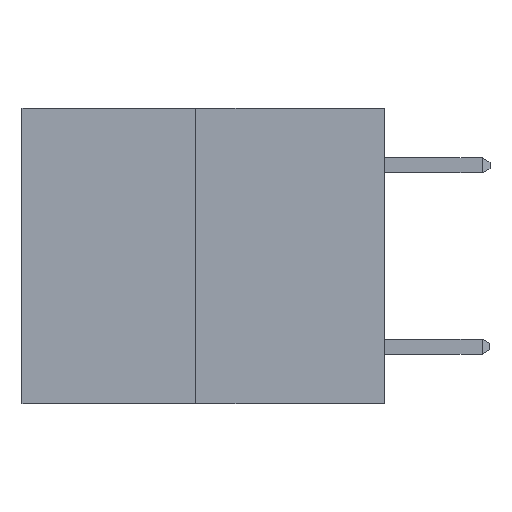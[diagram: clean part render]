
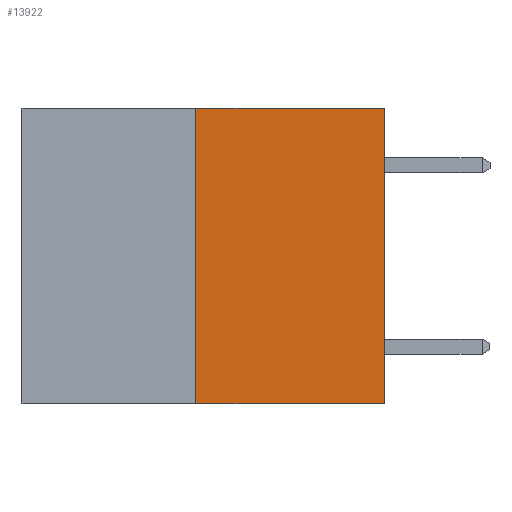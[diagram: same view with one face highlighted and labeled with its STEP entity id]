
A CAD part, left-side view. The second image highlights one B-rep face of the part: STEP entity #13922.
In plain terms, the highlighted planar face has unit normal (-1, 0, 0).
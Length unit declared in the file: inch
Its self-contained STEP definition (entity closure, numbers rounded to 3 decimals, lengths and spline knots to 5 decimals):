
#93 = DIRECTION ( 'NONE',  ( 0., -1., 0. ) ) ;
#161 = CARTESIAN_POINT ( 'NONE',  ( 0., 0.6, -0.49 ) ) ;
#312 = CARTESIAN_POINT ( 'NONE',  ( 0., 0., 0. ) ) ;
#816 = EDGE_CURVE ( 'NONE', #3410, #12007, #6694, .T. ) ;
#1347 = ORIENTED_EDGE ( 'NONE', *, *, #5956, .T. ) ;
#2114 = EDGE_CURVE ( 'NONE', #3410, #12522, #3185, .T. ) ;
#2272 = FACE_OUTER_BOUND ( 'NONE', #8951, .T. ) ;
#2341 = DIRECTION ( 'NONE',  ( 1., 0., 0. ) ) ;
#2649 = LINE ( 'NONE', #12723, #13413 ) ;
#2739 = ORIENTED_EDGE ( 'NONE', *, *, #816, .F. ) ;
#3018 = CARTESIAN_POINT ( 'NONE',  ( 0., 0.312, -0.49 ) ) ;
#3185 = LINE ( 'NONE', #161, #4123 ) ;
#3410 = VERTEX_POINT ( 'NONE', #3018 ) ;
#3694 = EDGE_CURVE ( 'NONE', #12007, #10917, #6509, .T. ) ;
#4123 = VECTOR ( 'NONE', #8460, 39.37008 ) ;
#5956 = EDGE_CURVE ( 'NONE', #12522, #10917, #2649, .T. ) ;
#6509 = LINE ( 'NONE', #13065, #11732 ) ;
#6694 = LINE ( 'NONE', #10881, #14350 ) ;
#7018 = PLANE ( 'NONE',  #8623 ) ;
#8460 = DIRECTION ( 'NONE',  ( 0., -1., 0. ) ) ;
#8578 = ORIENTED_EDGE ( 'NONE', *, *, #3694, .F. ) ;
#8623 = AXIS2_PLACEMENT_3D ( 'NONE', #9423, #2341, #10616 ) ;
#8951 = EDGE_LOOP ( 'NONE', ( #2739, #11652, #1347, #8578 ) ) ;
#9423 = CARTESIAN_POINT ( 'NONE',  ( 0., 0.6, 0. ) ) ;
#9550 = DIRECTION ( 'NONE',  ( 0., 0., 1. ) ) ;
#9712 = CARTESIAN_POINT ( 'NONE',  ( 0., 0., -0.49 ) ) ;
#10330 = CARTESIAN_POINT ( 'NONE',  ( 0., 0.312, 0. ) ) ;
#10531 = DIRECTION ( 'NONE',  ( 0., 0., 1. ) ) ;
#10616 = DIRECTION ( 'NONE',  ( 0., 0., -1. ) ) ;
#10881 = CARTESIAN_POINT ( 'NONE',  ( 0., 0.312, -0.49 ) ) ;
#10917 = VERTEX_POINT ( 'NONE', #312 ) ;
#11652 = ORIENTED_EDGE ( 'NONE', *, *, #2114, .T. ) ;
#11732 = VECTOR ( 'NONE', #93, 39.37008 ) ;
#12007 = VERTEX_POINT ( 'NONE', #10330 ) ;
#12522 = VERTEX_POINT ( 'NONE', #9712 ) ;
#12723 = CARTESIAN_POINT ( 'NONE',  ( 0., 0., 0. ) ) ;
#13065 = CARTESIAN_POINT ( 'NONE',  ( 0., 0.6, 0. ) ) ;
#13413 = VECTOR ( 'NONE', #10531, 39.37008 ) ;
#13922 = ADVANCED_FACE ( 'NONE', ( #2272 ), #7018, .F. ) ;
#14350 = VECTOR ( 'NONE', #9550, 39.37008 ) ;
